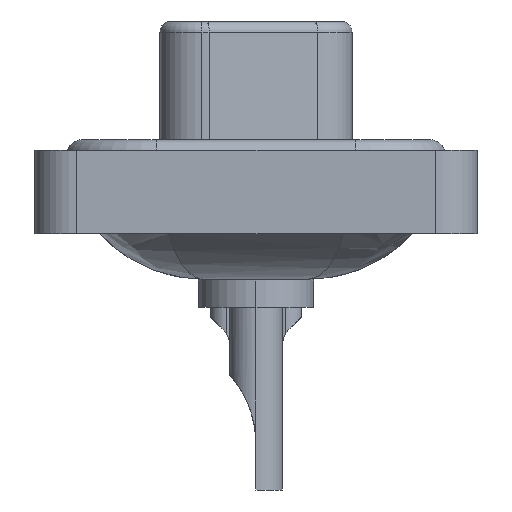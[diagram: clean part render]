
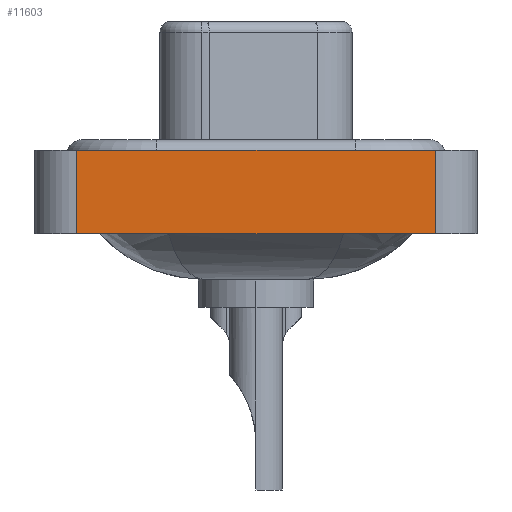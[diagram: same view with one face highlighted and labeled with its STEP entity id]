
A CAD part, left-side view. The second image highlights one B-rep face of the part: STEP entity #11603.
In plain terms, the highlighted planar face has unit normal (-1, 0, 0).
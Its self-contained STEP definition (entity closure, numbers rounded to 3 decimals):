
#615 = VECTOR ( 'NONE', #20093, 1000. ) ;
#3048 = VECTOR ( 'NONE', #11091, 1000. ) ;
#3179 = PLANE ( 'NONE',  #10494 ) ;
#3441 = CARTESIAN_POINT ( 'NONE',  ( -7.35, -8.55, -3.6 ) ) ;
#3723 = LINE ( 'NONE', #14436, #615 ) ;
#3918 = LINE ( 'NONE', #3441, #3048 ) ;
#4692 = VECTOR ( 'NONE', #5872, 1000. ) ;
#4765 = CARTESIAN_POINT ( 'NONE',  ( -7.35, -8.55, -3.6 ) ) ;
#5246 = EDGE_CURVE ( 'NONE', #19799, #13232, #9287, .T. ) ;
#5832 = DIRECTION ( 'NONE',  ( 0., -1., 0. ) ) ;
#5872 = DIRECTION ( 'NONE',  ( 0., -1., 0. ) ) ;
#9287 = LINE ( 'NONE', #16475, #4692 ) ;
#10258 = FACE_OUTER_BOUND ( 'NONE', #20629, .T. ) ;
#10494 = AXIS2_PLACEMENT_3D ( 'NONE', #15575, #14265, #17331 ) ;
#11091 = DIRECTION ( 'NONE',  ( 0., 0., 1. ) ) ;
#11341 = CARTESIAN_POINT ( 'NONE',  ( -7.35, -8.55, -3.6 ) ) ;
#11603 = ADVANCED_FACE ( 'NONE', ( #10258 ), #3179, .T. ) ;
#12948 = EDGE_CURVE ( 'NONE', #15360, #19799, #3723, .T. ) ;
#13232 = VERTEX_POINT ( 'NONE', #19245 ) ;
#13729 = LINE ( 'NONE', #4765, #14763 ) ;
#14265 = DIRECTION ( 'NONE',  ( -1., 0., 0. ) ) ;
#14436 = CARTESIAN_POINT ( 'NONE',  ( -7.35, 8.55, -3.6 ) ) ;
#14763 = VECTOR ( 'NONE', #5832, 1000. ) ;
#14782 = ORIENTED_EDGE ( 'NONE', *, *, #20444, .T. ) ;
#15360 = VERTEX_POINT ( 'NONE', #18246 ) ;
#15575 = CARTESIAN_POINT ( 'NONE',  ( -7.35, -8.55, -3.6 ) ) ;
#16431 = ORIENTED_EDGE ( 'NONE', *, *, #5246, .F. ) ;
#16475 = CARTESIAN_POINT ( 'NONE',  ( -7.35, -8.55, 0.4 ) ) ;
#17331 = DIRECTION ( 'NONE',  ( 0., 0., 1. ) ) ;
#17668 = VERTEX_POINT ( 'NONE', #11341 ) ;
#17683 = ORIENTED_EDGE ( 'NONE', *, *, #21097, .T. ) ;
#18246 = CARTESIAN_POINT ( 'NONE',  ( -7.35, 8.55, -3.6 ) ) ;
#18925 = CARTESIAN_POINT ( 'NONE',  ( -7.35, 8.55, 0.4 ) ) ;
#19245 = CARTESIAN_POINT ( 'NONE',  ( -7.35, -8.55, 0.4 ) ) ;
#19574 = ORIENTED_EDGE ( 'NONE', *, *, #12948, .F. ) ;
#19799 = VERTEX_POINT ( 'NONE', #18925 ) ;
#20093 = DIRECTION ( 'NONE',  ( 0., 0., 1. ) ) ;
#20444 = EDGE_CURVE ( 'NONE', #15360, #17668, #13729, .T. ) ;
#20629 = EDGE_LOOP ( 'NONE', ( #17683, #16431, #19574, #14782 ) ) ;
#21097 = EDGE_CURVE ( 'NONE', #17668, #13232, #3918, .T. ) ;
